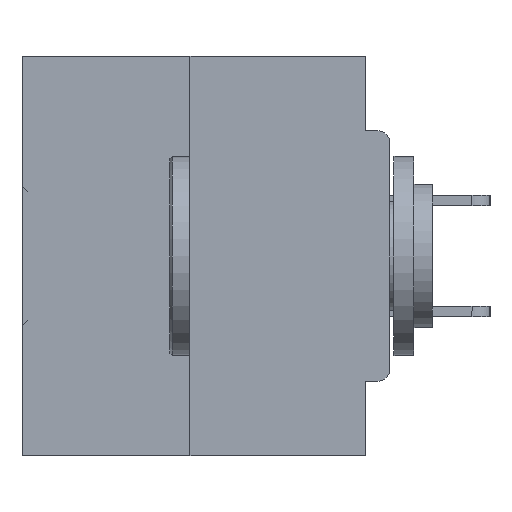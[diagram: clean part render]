
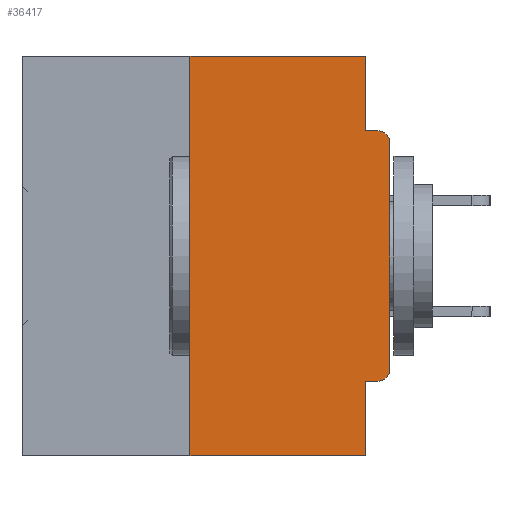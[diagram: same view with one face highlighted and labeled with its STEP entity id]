
A CAD part, left-side view. The second image highlights one B-rep face of the part: STEP entity #36417.
In plain terms, the highlighted planar face has unit normal (-1, 0, 0).
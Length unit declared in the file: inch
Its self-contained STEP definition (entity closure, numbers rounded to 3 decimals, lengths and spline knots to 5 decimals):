
#462 = ORIENTED_EDGE ( 'NONE', *, *, #47226, .F. ) ;
#1211 = AXIS2_PLACEMENT_3D ( 'NONE', #47068, #46431, #43175 ) ;
#1240 = CARTESIAN_POINT ( 'NONE',  ( 0., 0.46, 0. ) ) ;
#3141 = CARTESIAN_POINT ( 'NONE',  ( 0., 0.46, -0.5 ) ) ;
#3479 = VERTEX_POINT ( 'NONE', #27050 ) ;
#3692 = CARTESIAN_POINT ( 'NONE',  ( 0., 0.031, -0.5 ) ) ;
#3899 = VECTOR ( 'NONE', #43705, 39.37008 ) ;
#4180 = ORIENTED_EDGE ( 'NONE', *, *, #8276, .F. ) ;
#4465 = EDGE_CURVE ( 'NONE', #7344, #45155, #25424, .T. ) ;
#4957 = AXIS2_PLACEMENT_3D ( 'NONE', #16767, #38775, #5876 ) ;
#5040 = LINE ( 'NONE', #3141, #3899 ) ;
#5734 = DIRECTION ( 'NONE',  ( 0., 1., 0. ) ) ;
#5876 = DIRECTION ( 'NONE',  ( 0., 0., -1. ) ) ;
#5915 = VECTOR ( 'NONE', #13761, 39.37008 ) ;
#6088 = CARTESIAN_POINT ( 'NONE',  ( 0., 0., 0. ) ) ;
#6522 = DIRECTION ( 'NONE',  ( 1., 0., 0. ) ) ;
#6758 = CARTESIAN_POINT ( 'NONE',  ( 0., 0.031, 0. ) ) ;
#7344 = VERTEX_POINT ( 'NONE', #10503 ) ;
#8230 = VERTEX_POINT ( 'NONE', #34248 ) ;
#8276 = EDGE_CURVE ( 'NONE', #38086, #21596, #10116, .T. ) ;
#9588 = PLANE ( 'NONE',  #24427 ) ;
#10116 = LINE ( 'NONE', #22090, #36964 ) ;
#10271 = VERTEX_POINT ( 'NONE', #43759 ) ;
#10337 = CARTESIAN_POINT ( 'NONE',  ( 0., 0.25, 0. ) ) ;
#10415 = CIRCLE ( 'NONE', #1211, 0.015 ) ;
#10503 = CARTESIAN_POINT ( 'NONE',  ( 0., 0.031, 0. ) ) ;
#10575 = EDGE_CURVE ( 'NONE', #11780, #38086, #34009, .T. ) ;
#10584 = EDGE_CURVE ( 'NONE', #45155, #8230, #22591, .T. ) ;
#11586 = EDGE_CURVE ( 'NONE', #11780, #10271, #16144, .T. ) ;
#11780 = VERTEX_POINT ( 'NONE', #43496 ) ;
#12255 = FACE_OUTER_BOUND ( 'NONE', #46804, .T. ) ;
#12448 = CARTESIAN_POINT ( 'NONE',  ( 0., 0., -0.1085 ) ) ;
#13761 = DIRECTION ( 'NONE',  ( 0., 0., -1. ) ) ;
#15767 = EDGE_CURVE ( 'NONE', #29915, #21596, #5040, .T. ) ;
#16144 = CIRCLE ( 'NONE', #4957, 0.015 ) ;
#16767 = CARTESIAN_POINT ( 'NONE',  ( 0., 0.015, -0.3915 ) ) ;
#16932 = DIRECTION ( 'NONE',  ( 0., -1., 0. ) ) ;
#17404 = CARTESIAN_POINT ( 'NONE',  ( 0., 0.46, 0. ) ) ;
#20148 = ORIENTED_EDGE ( 'NONE', *, *, #37564, .F. ) ;
#20495 = DIRECTION ( 'NONE',  ( 0., 0., 1. ) ) ;
#20779 = VECTOR ( 'NONE', #43037, 39.37008 ) ;
#21450 = VECTOR ( 'NONE', #16932, 39.37008 ) ;
#21596 = VERTEX_POINT ( 'NONE', #3692 ) ;
#21800 = ORIENTED_EDGE ( 'NONE', *, *, #30167, .T. ) ;
#22090 = CARTESIAN_POINT ( 'NONE',  ( 0., 0.031, -0.5 ) ) ;
#22591 = LINE ( 'NONE', #31357, #21450 ) ;
#23139 = CARTESIAN_POINT ( 'NONE',  ( 0., 0.25, -0.5 ) ) ;
#23163 = ORIENTED_EDGE ( 'NONE', *, *, #4465, .F. ) ;
#23313 = VECTOR ( 'NONE', #34032, 39.37008 ) ;
#24307 = DIRECTION ( 'NONE',  ( 0., 0., -1. ) ) ;
#24427 = AXIS2_PLACEMENT_3D ( 'NONE', #17404, #6522, #24307 ) ;
#24732 = ORIENTED_EDGE ( 'NONE', *, *, #10584, .F. ) ;
#25424 = LINE ( 'NONE', #6758, #5915 ) ;
#26188 = ORIENTED_EDGE ( 'NONE', *, *, #46733, .T. ) ;
#26396 = CARTESIAN_POINT ( 'NONE',  ( 0., 0.031, -0.0935 ) ) ;
#26606 = VECTOR ( 'NONE', #5734, 39.37008 ) ;
#27050 = CARTESIAN_POINT ( 'NONE',  ( 0., 0.25, 0. ) ) ;
#27972 = VECTOR ( 'NONE', #20495, 39.37008 ) ;
#29915 = VERTEX_POINT ( 'NONE', #23139 ) ;
#30167 = EDGE_CURVE ( 'NONE', #36303, #8230, #10415, .T. ) ;
#31357 = CARTESIAN_POINT ( 'NONE',  ( 0., 0., -0.0935 ) ) ;
#32784 = LINE ( 'NONE', #10337, #20779 ) ;
#32794 = DIRECTION ( 'NONE',  ( 0., 0., -1. ) ) ;
#34009 = LINE ( 'NONE', #38941, #26606 ) ;
#34032 = DIRECTION ( 'NONE',  ( 0., -1., 0. ) ) ;
#34248 = CARTESIAN_POINT ( 'NONE',  ( 0., 0.015, -0.0935 ) ) ;
#34559 = ORIENTED_EDGE ( 'NONE', *, *, #15767, .T. ) ;
#35697 = ORIENTED_EDGE ( 'NONE', *, *, #11586, .T. ) ;
#36303 = VERTEX_POINT ( 'NONE', #12448 ) ;
#36417 = ADVANCED_FACE ( 'NONE', ( #12255 ), #9588, .F. ) ;
#36964 = VECTOR ( 'NONE', #32794, 39.37008 ) ;
#37564 = EDGE_CURVE ( 'NONE', #29915, #3479, #32784, .T. ) ;
#38086 = VERTEX_POINT ( 'NONE', #40139 ) ;
#38775 = DIRECTION ( 'NONE',  ( -1., 0., 0. ) ) ;
#38941 = CARTESIAN_POINT ( 'NONE',  ( 0., 0., -0.4065 ) ) ;
#40139 = CARTESIAN_POINT ( 'NONE',  ( 0., 0.031, -0.4065 ) ) ;
#42189 = LINE ( 'NONE', #6088, #27972 ) ;
#43037 = DIRECTION ( 'NONE',  ( 0., 0., 1. ) ) ;
#43175 = DIRECTION ( 'NONE',  ( 0., 0., -1. ) ) ;
#43496 = CARTESIAN_POINT ( 'NONE',  ( 0., 0.015, -0.4065 ) ) ;
#43705 = DIRECTION ( 'NONE',  ( 0., -1., 0. ) ) ;
#43759 = CARTESIAN_POINT ( 'NONE',  ( 0., 0., -0.3915 ) ) ;
#44768 = ORIENTED_EDGE ( 'NONE', *, *, #10575, .F. ) ;
#45155 = VERTEX_POINT ( 'NONE', #26396 ) ;
#45549 = LINE ( 'NONE', #1240, #23313 ) ;
#46431 = DIRECTION ( 'NONE',  ( -1., 0., 0. ) ) ;
#46733 = EDGE_CURVE ( 'NONE', #10271, #36303, #42189, .T. ) ;
#46804 = EDGE_LOOP ( 'NONE', ( #462, #20148, #34559, #4180, #44768, #35697, #26188, #21800, #24732, #23163 ) ) ;
#47068 = CARTESIAN_POINT ( 'NONE',  ( 0., 0.015, -0.1085 ) ) ;
#47226 = EDGE_CURVE ( 'NONE', #3479, #7344, #45549, .T. ) ;
